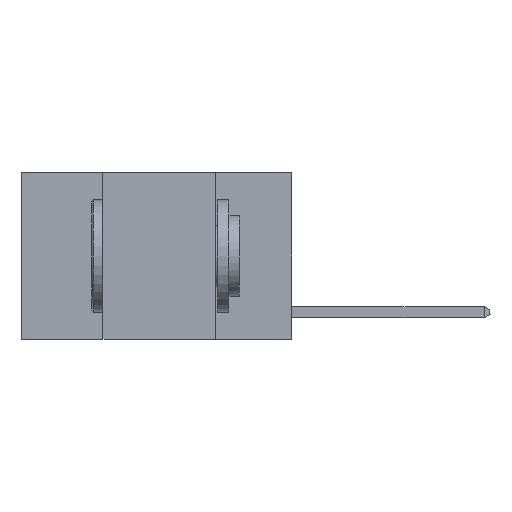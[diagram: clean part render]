
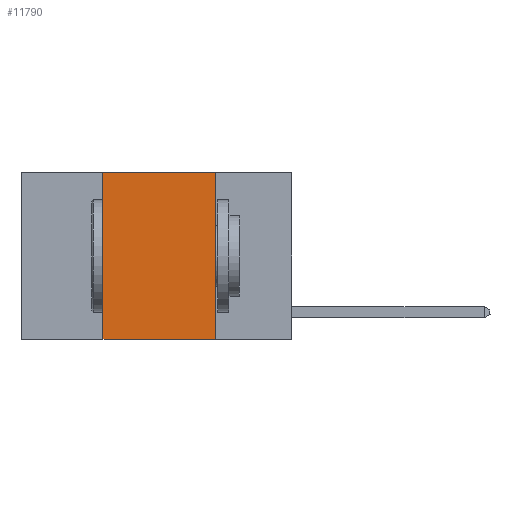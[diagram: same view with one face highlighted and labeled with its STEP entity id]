
A CAD part, left-side view. The second image highlights one B-rep face of the part: STEP entity #11790.
In plain terms, the highlighted planar face has unit normal (-1, 0, 0).
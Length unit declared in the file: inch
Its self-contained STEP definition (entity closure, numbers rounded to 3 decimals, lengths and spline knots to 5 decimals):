
#204 = DIRECTION ( 'NONE',  ( 0., 0., 1. ) ) ;
#1090 = VECTOR ( 'NONE', #7379, 39.37008 ) ;
#1572 = ORIENTED_EDGE ( 'NONE', *, *, #13458, .T. ) ;
#1890 = VERTEX_POINT ( 'NONE', #9040 ) ;
#2120 = PLANE ( 'NONE',  #13660 ) ;
#2235 = EDGE_CURVE ( 'NONE', #9331, #11446, #4567, .T. ) ;
#2246 = DIRECTION ( 'NONE',  ( 0., -1., 0. ) ) ;
#2485 = CARTESIAN_POINT ( 'NONE',  ( 0., 0.17, 0. ) ) ;
#3098 = EDGE_LOOP ( 'NONE', ( #4711, #9837, #5438, #1572 ) ) ;
#3178 = FACE_OUTER_BOUND ( 'NONE', #3098, .T. ) ;
#4467 = CARTESIAN_POINT ( 'NONE',  ( 0., 0.6, 0. ) ) ;
#4567 = LINE ( 'NONE', #2485, #7163 ) ;
#4711 = ORIENTED_EDGE ( 'NONE', *, *, #2235, .F. ) ;
#5295 = LINE ( 'NONE', #9513, #1090 ) ;
#5438 = ORIENTED_EDGE ( 'NONE', *, *, #7338, .F. ) ;
#5651 = LINE ( 'NONE', #9891, #11372 ) ;
#6348 = EDGE_CURVE ( 'NONE', #6940, #9331, #9457, .T. ) ;
#6940 = VERTEX_POINT ( 'NONE', #11867 ) ;
#7163 = VECTOR ( 'NONE', #7969, 39.37008 ) ;
#7338 = EDGE_CURVE ( 'NONE', #1890, #6940, #5651, .T. ) ;
#7379 = DIRECTION ( 'NONE',  ( 0., -1., 0. ) ) ;
#7969 = DIRECTION ( 'NONE',  ( 0., 0., -1. ) ) ;
#8050 = CARTESIAN_POINT ( 'NONE',  ( 0., 0.17, -0.37 ) ) ;
#8523 = CARTESIAN_POINT ( 'NONE',  ( 0., 0.6, 0. ) ) ;
#9040 = CARTESIAN_POINT ( 'NONE',  ( 0., 0.42, -0.37 ) ) ;
#9331 = VERTEX_POINT ( 'NONE', #9746 ) ;
#9457 = LINE ( 'NONE', #4467, #13351 ) ;
#9513 = CARTESIAN_POINT ( 'NONE',  ( 0., 0.6, -0.37 ) ) ;
#9746 = CARTESIAN_POINT ( 'NONE',  ( 0., 0.17, 0. ) ) ;
#9837 = ORIENTED_EDGE ( 'NONE', *, *, #6348, .F. ) ;
#9880 = DIRECTION ( 'NONE',  ( 0., 0., -1. ) ) ;
#9891 = CARTESIAN_POINT ( 'NONE',  ( 0., 0.42, 0. ) ) ;
#10987 = DIRECTION ( 'NONE',  ( 1., 0., 0. ) ) ;
#11372 = VECTOR ( 'NONE', #204, 39.37008 ) ;
#11446 = VERTEX_POINT ( 'NONE', #8050 ) ;
#11790 = ADVANCED_FACE ( 'NONE', ( #3178 ), #2120, .F. ) ;
#11867 = CARTESIAN_POINT ( 'NONE',  ( 0., 0.42, 0. ) ) ;
#13351 = VECTOR ( 'NONE', #2246, 39.37008 ) ;
#13458 = EDGE_CURVE ( 'NONE', #1890, #11446, #5295, .T. ) ;
#13660 = AXIS2_PLACEMENT_3D ( 'NONE', #8523, #10987, #9880 ) ;
